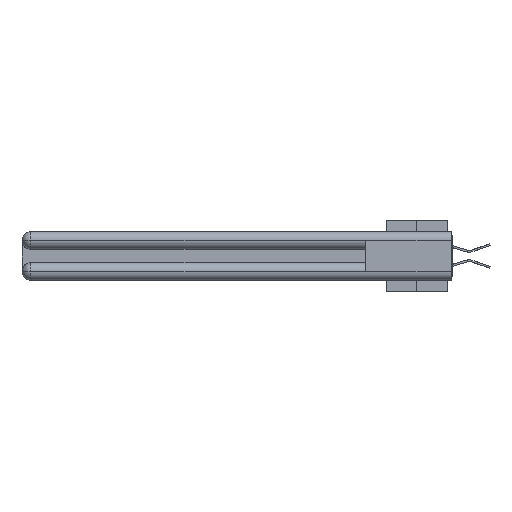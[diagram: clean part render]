
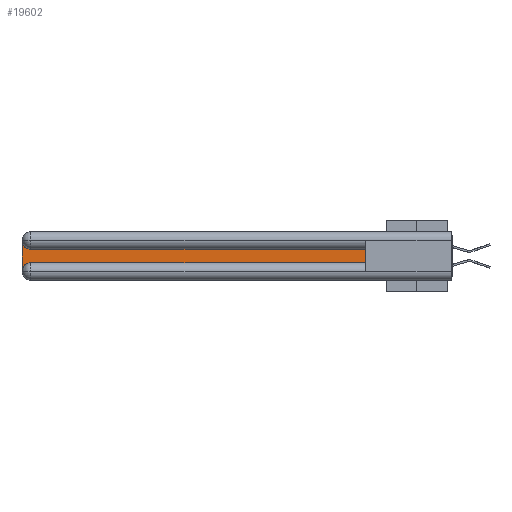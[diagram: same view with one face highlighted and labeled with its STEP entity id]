
A CAD part, left-side view. The second image highlights one B-rep face of the part: STEP entity #19602.
In plain terms, the highlighted planar face has unit normal (-1, 0, 0).
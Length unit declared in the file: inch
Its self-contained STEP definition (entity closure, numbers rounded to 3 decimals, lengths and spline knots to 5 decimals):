
#210 = LINE ( 'NONE', #4820, #31608 ) ;
#928 = CARTESIAN_POINT ( 'NONE',  ( 0.075, 3., -0.1225 ) ) ;
#1097 = ORIENTED_EDGE ( 'NONE', *, *, #19082, .T. ) ;
#4820 = CARTESIAN_POINT ( 'NONE',  ( 0.075, 0.6, -0.1225 ) ) ;
#5324 = EDGE_CURVE ( 'NONE', #10204, #27787, #18735, .T. ) ;
#6315 = DIRECTION ( 'NONE',  ( 0., 0., -1. ) ) ;
#6577 = EDGE_CURVE ( 'NONE', #22007, #22173, #25843, .T. ) ;
#6995 = ORIENTED_EDGE ( 'NONE', *, *, #20406, .T. ) ;
#7598 = CARTESIAN_POINT ( 'NONE',  ( 0.075, 3., -0.0625 ) ) ;
#8618 = VERTEX_POINT ( 'NONE', #27690 ) ;
#9018 = CARTESIAN_POINT ( 'NONE',  ( 0.075, 0.6, -0.1225 ) ) ;
#10204 = VERTEX_POINT ( 'NONE', #7598 ) ;
#10748 = CARTESIAN_POINT ( 'NONE',  ( 0.075, 2.94, -0.2175 ) ) ;
#13144 = EDGE_CURVE ( 'NONE', #8618, #10204, #19392, .T. ) ;
#13350 = CIRCLE ( 'NONE', #28259, 0.06 ) ;
#14341 = DIRECTION ( 'NONE',  ( 0., 1., 0. ) ) ;
#15233 = FACE_OUTER_BOUND ( 'NONE', #23276, .T. ) ;
#16235 = ORIENTED_EDGE ( 'NONE', *, *, #28559, .T. ) ;
#16906 = ORIENTED_EDGE ( 'NONE', *, *, #13144, .T. ) ;
#17516 = CARTESIAN_POINT ( 'NONE',  ( 0.075, 0.6, -0.2175 ) ) ;
#18150 = VECTOR ( 'NONE', #24616, 39.37008 ) ;
#18472 = CARTESIAN_POINT ( 'NONE',  ( 0.075, 3., -0.2775 ) ) ;
#18735 = LINE ( 'NONE', #26077, #21631 ) ;
#19082 = EDGE_CURVE ( 'NONE', #26526, #22007, #38075, .T. ) ;
#19174 = DIRECTION ( 'NONE',  ( 1., 0., 0. ) ) ;
#19392 = CIRCLE ( 'NONE', #32918, 0.06 ) ;
#19602 = ADVANCED_FACE ( 'NONE', ( #15233 ), #34631, .F. ) ;
#20406 = EDGE_CURVE ( 'NONE', #22173, #8618, #210, .T. ) ;
#21196 = DIRECTION ( 'NONE',  ( 0., 0., -1. ) ) ;
#21275 = CARTESIAN_POINT ( 'NONE',  ( 0.075, 2.94, -0.0625 ) ) ;
#21631 = VECTOR ( 'NONE', #35754, 39.37008 ) ;
#22007 = VERTEX_POINT ( 'NONE', #17516 ) ;
#22173 = VERTEX_POINT ( 'NONE', #9018 ) ;
#23276 = EDGE_LOOP ( 'NONE', ( #6995, #16906, #29744, #16235, #1097, #27847 ) ) ;
#24616 = DIRECTION ( 'NONE',  ( 0., 0., 1. ) ) ;
#25843 = LINE ( 'NONE', #39942, #18150 ) ;
#26077 = CARTESIAN_POINT ( 'NONE',  ( 0.075, 3., -0.2175 ) ) ;
#26526 = VERTEX_POINT ( 'NONE', #10748 ) ;
#27690 = CARTESIAN_POINT ( 'NONE',  ( 0.075, 2.94, -0.1225 ) ) ;
#27787 = VERTEX_POINT ( 'NONE', #18472 ) ;
#27847 = ORIENTED_EDGE ( 'NONE', *, *, #6577, .T. ) ;
#28259 = AXIS2_PLACEMENT_3D ( 'NONE', #32992, #29867, #21196 ) ;
#28559 = EDGE_CURVE ( 'NONE', #27787, #26526, #13350, .T. ) ;
#29518 = DIRECTION ( 'NONE',  ( 0., -1., 0. ) ) ;
#29744 = ORIENTED_EDGE ( 'NONE', *, *, #5324, .T. ) ;
#29867 = DIRECTION ( 'NONE',  ( 1., 0., 0. ) ) ;
#30888 = DIRECTION ( 'NONE',  ( 1., 0., 0. ) ) ;
#31245 = AXIS2_PLACEMENT_3D ( 'NONE', #928, #19174, #37469 ) ;
#31608 = VECTOR ( 'NONE', #14341, 39.37008 ) ;
#32101 = CARTESIAN_POINT ( 'NONE',  ( 0.075, 0.6, -0.2175 ) ) ;
#32918 = AXIS2_PLACEMENT_3D ( 'NONE', #21275, #30888, #6315 ) ;
#32992 = CARTESIAN_POINT ( 'NONE',  ( 0.075, 2.94, -0.2775 ) ) ;
#34631 = PLANE ( 'NONE',  #31245 ) ;
#35754 = DIRECTION ( 'NONE',  ( 0., 0., -1. ) ) ;
#36659 = VECTOR ( 'NONE', #29518, 39.37008 ) ;
#37469 = DIRECTION ( 'NONE',  ( 0., 0., -1. ) ) ;
#38075 = LINE ( 'NONE', #32101, #36659 ) ;
#39942 = CARTESIAN_POINT ( 'NONE',  ( 0.075, 0.6, -0.2175 ) ) ;
